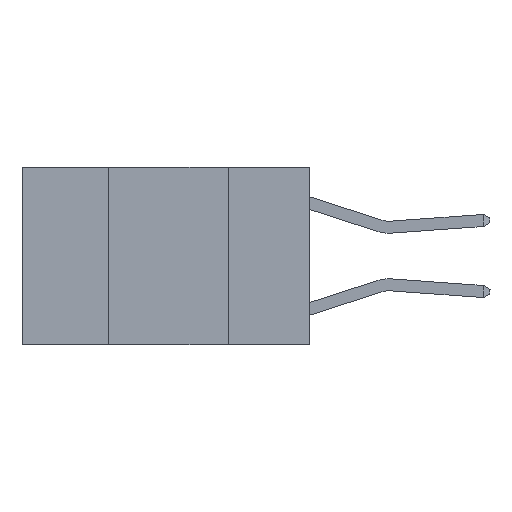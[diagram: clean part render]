
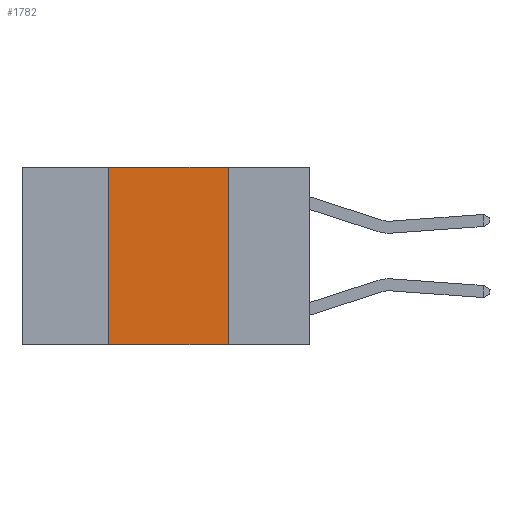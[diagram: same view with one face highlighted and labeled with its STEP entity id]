
A CAD part, left-side view. The second image highlights one B-rep face of the part: STEP entity #1782.
In plain terms, the highlighted planar face has unit normal (-1, 0, 0).
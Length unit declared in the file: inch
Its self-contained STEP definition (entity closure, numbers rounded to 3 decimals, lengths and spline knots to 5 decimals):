
#449 = CARTESIAN_POINT ( 'NONE',  ( 0., 0.42, 0. ) ) ;
#1213 = AXIS2_PLACEMENT_3D ( 'NONE', #8905, #22242, #10811 ) ;
#1782 = ADVANCED_FACE ( 'NONE', ( #10667 ), #20360, .F. ) ;
#2057 = VERTEX_POINT ( 'NONE', #5842 ) ;
#3538 = VECTOR ( 'NONE', #19575, 39.37008 ) ;
#4928 = DIRECTION ( 'NONE',  ( 0., -1., 0. ) ) ;
#5666 = CARTESIAN_POINT ( 'NONE',  ( 0., 0.42, -0.37 ) ) ;
#5777 = VECTOR ( 'NONE', #4928, 39.37008 ) ;
#5842 = CARTESIAN_POINT ( 'NONE',  ( 0., 0.42, 0. ) ) ;
#6319 = VERTEX_POINT ( 'NONE', #5666 ) ;
#7276 = EDGE_CURVE ( 'NONE', #15113, #12272, #22512, .T. ) ;
#8162 = ORIENTED_EDGE ( 'NONE', *, *, #17658, .F. ) ;
#8905 = CARTESIAN_POINT ( 'NONE',  ( 0., 0.6, 0. ) ) ;
#9344 = ORIENTED_EDGE ( 'NONE', *, *, #13641, .T. ) ;
#9821 = EDGE_CURVE ( 'NONE', #6319, #2057, #19367, .T. ) ;
#10226 = CARTESIAN_POINT ( 'NONE',  ( 0., 0.17, -0.37 ) ) ;
#10667 = FACE_OUTER_BOUND ( 'NONE', #20486, .T. ) ;
#10807 = LINE ( 'NONE', #22088, #5777 ) ;
#10811 = DIRECTION ( 'NONE',  ( 0., 0., -1. ) ) ;
#12272 = VERTEX_POINT ( 'NONE', #10226 ) ;
#13641 = EDGE_CURVE ( 'NONE', #6319, #12272, #10807, .T. ) ;
#15113 = VERTEX_POINT ( 'NONE', #20596 ) ;
#15632 = DIRECTION ( 'NONE',  ( 0., 0., -1. ) ) ;
#15883 = CARTESIAN_POINT ( 'NONE',  ( 0., 0.17, 0. ) ) ;
#17658 = EDGE_CURVE ( 'NONE', #2057, #15113, #22757, .T. ) ;
#17718 = VECTOR ( 'NONE', #20238, 39.37008 ) ;
#17728 = ORIENTED_EDGE ( 'NONE', *, *, #7276, .F. ) ;
#18921 = ORIENTED_EDGE ( 'NONE', *, *, #9821, .F. ) ;
#19367 = LINE ( 'NONE', #449, #3538 ) ;
#19575 = DIRECTION ( 'NONE',  ( 0., 0., 1. ) ) ;
#20238 = DIRECTION ( 'NONE',  ( 0., -1., 0. ) ) ;
#20360 = PLANE ( 'NONE',  #1213 ) ;
#20486 = EDGE_LOOP ( 'NONE', ( #17728, #8162, #18921, #9344 ) ) ;
#20596 = CARTESIAN_POINT ( 'NONE',  ( 0., 0.17, 0. ) ) ;
#21913 = VECTOR ( 'NONE', #15632, 39.37008 ) ;
#22088 = CARTESIAN_POINT ( 'NONE',  ( 0., 0.6, -0.37 ) ) ;
#22242 = DIRECTION ( 'NONE',  ( 1., 0., 0. ) ) ;
#22512 = LINE ( 'NONE', #15883, #21913 ) ;
#22757 = LINE ( 'NONE', #23955, #17718 ) ;
#23955 = CARTESIAN_POINT ( 'NONE',  ( 0., 0.6, 0. ) ) ;
